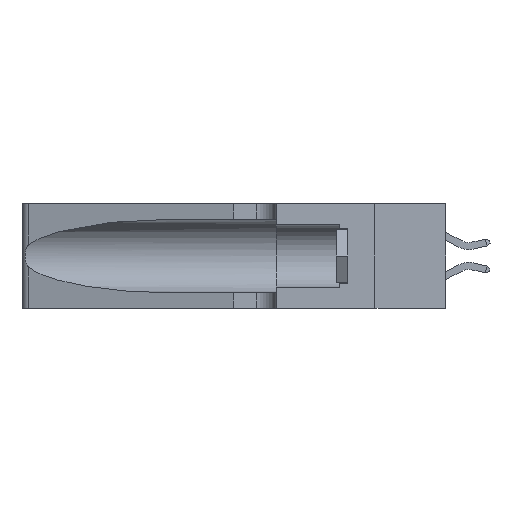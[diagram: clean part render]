
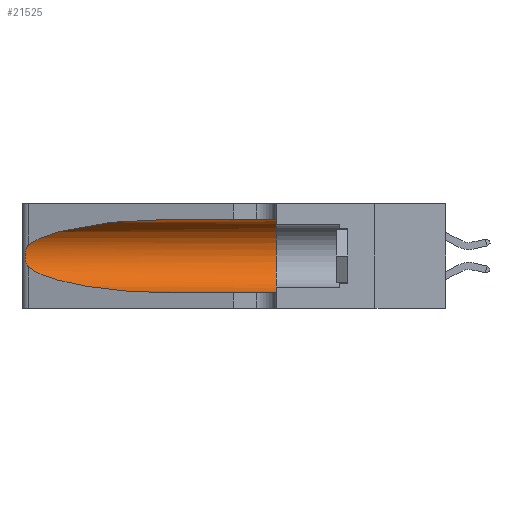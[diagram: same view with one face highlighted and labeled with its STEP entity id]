
A CAD part, left-side view. The second image highlights one B-rep face of the part: STEP entity #21525.
In plain terms, the highlighted cylindrical face has radius 3.308 mm (diameter 6.617 mm), a partial arc.
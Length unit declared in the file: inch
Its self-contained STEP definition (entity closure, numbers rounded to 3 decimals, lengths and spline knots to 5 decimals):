
#243 =( BOUNDED_CURVE ( )  B_SPLINE_CURVE ( 3, ( #1837, #3470, #8435, #13591 ),
 .UNSPECIFIED., .F., .F. ) 
 B_SPLINE_CURVE_WITH_KNOTS ( ( 4, 4 ),
 ( 1.5708, 2.84003 ),
 .UNSPECIFIED. ) 
 CURVE ( )  GEOMETRIC_REPRESENTATION_ITEM ( )  RATIONAL_B_SPLINE_CURVE ( ( 1., 0.87, 0.87, 1. ) ) 
 REPRESENTATION_ITEM ( '' )  );
#615 = VECTOR ( 'NONE', #9088, 39.37008 ) ;
#646 = EDGE_CURVE ( 'NONE', #19099, #18617, #13553, .T. ) ;
#662 = VERTEX_POINT ( 'NONE', #18703 ) ;
#1154 = DIRECTION ( 'NONE',  ( 0., -1., 0. ) ) ;
#1598 = EDGE_LOOP ( 'NONE', ( #1815, #6030, #14997, #19562, #16798, #14425 ) ) ;
#1815 = ORIENTED_EDGE ( 'NONE', *, *, #8347, .T. ) ;
#1837 = CARTESIAN_POINT ( 'NONE',  ( 0.1305, 0.72297, 0.31525 ) ) ;
#2036 = EDGE_CURVE ( 'NONE', #2635, #662, #13472, .T. ) ;
#2618 = CARTESIAN_POINT ( 'NONE',  ( 0.1305, 0.72297, 0.31525 ) ) ;
#2635 = VERTEX_POINT ( 'NONE', #8352 ) ;
#3470 = CARTESIAN_POINT ( 'NONE',  ( 0.18966, 0.96281, 0.31525 ) ) ;
#3882 = LINE ( 'NONE', #11196, #15990 ) ;
#4337 = EDGE_CURVE ( 'NONE', #20349, #2635, #17435, .T. ) ;
#4604 = FACE_OUTER_BOUND ( 'NONE', #1598, .T. ) ;
#5001 = DIRECTION ( 'NONE',  ( 0., 1., 0. ) ) ;
#5584 = CARTESIAN_POINT ( 'NONE',  ( 0.26075, 1.23896, 0.178 ) ) ;
#6030 = ORIENTED_EDGE ( 'NONE', *, *, #11343, .T. ) ;
#6124 = AXIS2_PLACEMENT_3D ( 'NONE', #6961, #15790, #15871 ) ;
#6238 = VERTEX_POINT ( 'NONE', #8850 ) ;
#6377 = CARTESIAN_POINT ( 'NONE',  ( 0.25487, 1.22718, 0.14631 ) ) ;
#6685 = CARTESIAN_POINT ( 'NONE',  ( 0.1305, 0.72297, 0.05475 ) ) ;
#6961 = CARTESIAN_POINT ( 'NONE',  ( 0.1305, 1.61858, 0.185 ) ) ;
#8347 = EDGE_CURVE ( 'NONE', #20349, #6238, #243, .T. ) ;
#8352 = CARTESIAN_POINT ( 'NONE',  ( 0.1305, 0.35, 0.31525 ) ) ;
#8435 = CARTESIAN_POINT ( 'NONE',  ( 0.2373, 1.15595, 0.28018 ) ) ;
#8822 = CARTESIAN_POINT ( 'NONE',  ( 0.26017, 1.23833, 0.17102 ) ) ;
#8850 = CARTESIAN_POINT ( 'NONE',  ( 0.25487, 1.22718, 0.22369 ) ) ;
#8892 = CARTESIAN_POINT ( 'NONE',  ( 0.25789, 1.23486, 0.15765 ) ) ;
#9050 = CARTESIAN_POINT ( 'NONE',  ( 0.26075, 1.23896, 0.19203 ) ) ;
#9088 = DIRECTION ( 'NONE',  ( 0., -1., 0. ) ) ;
#10474 = CARTESIAN_POINT ( 'NONE',  ( 0.1305, 0.72297, 0.05475 ) ) ;
#10671 = CARTESIAN_POINT ( 'NONE',  ( 0.25487, 1.22718, 0.14631 ) ) ;
#10741 = CARTESIAN_POINT ( 'NONE',  ( 0.25787, 1.23484, 0.2124 ) ) ;
#11196 = CARTESIAN_POINT ( 'NONE',  ( 0.1305, 1.61858, 0.05475 ) ) ;
#11343 = EDGE_CURVE ( 'NONE', #6238, #19099, #20413, .T. ) ;
#13472 = CIRCLE ( 'NONE', #17061, 0.13025 ) ;
#13553 =( BOUNDED_CURVE ( )  B_SPLINE_CURVE ( 3, ( #17151, #20394, #15491, #10474 ),
 .UNSPECIFIED., .F., .F. ) 
 B_SPLINE_CURVE_WITH_KNOTS ( ( 4, 4 ),
 ( 3.44316, 4.71239 ),
 .UNSPECIFIED. ) 
 CURVE ( )  GEOMETRIC_REPRESENTATION_ITEM ( )  RATIONAL_B_SPLINE_CURVE ( ( 1., 0.87, 0.87, 1. ) ) 
 REPRESENTATION_ITEM ( '' )  );
#13591 = CARTESIAN_POINT ( 'NONE',  ( 0.25487, 1.22718, 0.22369 ) ) ;
#13681 = CARTESIAN_POINT ( 'NONE',  ( 0.1305, 0.35, 0.185 ) ) ;
#13829 = CARTESIAN_POINT ( 'NONE',  ( 0.25487, 1.22718, 0.22369 ) ) ;
#14055 = CARTESIAN_POINT ( 'NONE',  ( 0.25639, 1.23184, 0.21858 ) ) ;
#14117 = CARTESIAN_POINT ( 'NONE',  ( 0.25555, 1.22993, 0.14849 ) ) ;
#14425 = ORIENTED_EDGE ( 'NONE', *, *, #4337, .F. ) ;
#14997 = ORIENTED_EDGE ( 'NONE', *, *, #646, .T. ) ;
#15222 = EDGE_CURVE ( 'NONE', #18617, #662, #3882, .T. ) ;
#15491 = CARTESIAN_POINT ( 'NONE',  ( 0.18966, 0.96281, 0.05475 ) ) ;
#15743 = CARTESIAN_POINT ( 'NONE',  ( 0.26018, 1.23835, 0.19895 ) ) ;
#15790 = DIRECTION ( 'NONE',  ( 0., -1., 0. ) ) ;
#15871 = DIRECTION ( 'NONE',  ( 0., 0., -1. ) ) ;
#15990 = VECTOR ( 'NONE', #1154, 39.37008 ) ;
#16776 = DIRECTION ( 'NONE',  ( 0., 0., 1. ) ) ;
#16798 = ORIENTED_EDGE ( 'NONE', *, *, #2036, .F. ) ;
#17061 = AXIS2_PLACEMENT_3D ( 'NONE', #13681, #5001, #16776 ) ;
#17151 = CARTESIAN_POINT ( 'NONE',  ( 0.25487, 1.22718, 0.14631 ) ) ;
#17435 = LINE ( 'NONE', #17476, #615 ) ;
#17476 = CARTESIAN_POINT ( 'NONE',  ( 0.1305, 1.61858, 0.31525 ) ) ;
#18570 = CYLINDRICAL_SURFACE ( 'NONE', #6124, 0.13025 ) ;
#18617 = VERTEX_POINT ( 'NONE', #6685 ) ;
#18703 = CARTESIAN_POINT ( 'NONE',  ( 0.1305, 0.35, 0.05475 ) ) ;
#18899 = CARTESIAN_POINT ( 'NONE',  ( 0.25854, 1.2359, 0.20912 ) ) ;
#18979 = CARTESIAN_POINT ( 'NONE',  ( 0.25555, 1.22994, 0.2215 ) ) ;
#19099 = VERTEX_POINT ( 'NONE', #6377 ) ;
#19562 = ORIENTED_EDGE ( 'NONE', *, *, #15222, .T. ) ;
#20349 = VERTEX_POINT ( 'NONE', #2618 ) ;
#20394 = CARTESIAN_POINT ( 'NONE',  ( 0.2373, 1.15595, 0.08982 ) ) ;
#20413 = B_SPLINE_CURVE_WITH_KNOTS ( 'NONE', 3,
 ( #13829, #18979, #14055, #10741, #18899, #15743, #9050, #5584, #8822, #20583, #8892, #20661, #14117, #10671 ),
 .UNSPECIFIED., .F., .F.,
 ( 4, 2, 2, 2, 2, 2, 4 ),
 ( 0., 0.00027, 0.00053, 0.00107, 0.0016, 0.00187, 0.00214 ),
 .UNSPECIFIED. ) ;
#20583 = CARTESIAN_POINT ( 'NONE',  ( 0.25856, 1.23593, 0.16098 ) ) ;
#20661 = CARTESIAN_POINT ( 'NONE',  ( 0.25639, 1.23186, 0.15144 ) ) ;
#21525 = ADVANCED_FACE ( 'NONE', ( #4604 ), #18570, .F. ) ;
